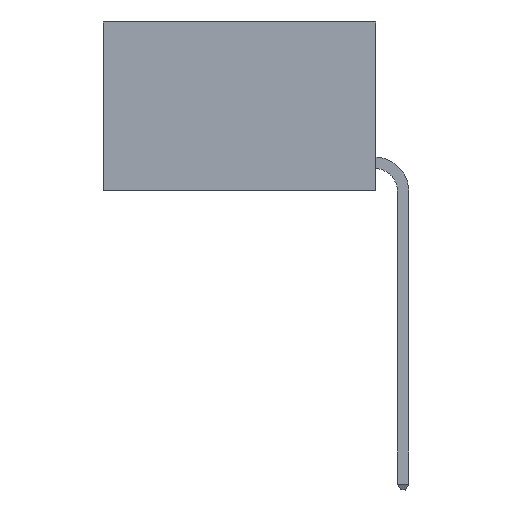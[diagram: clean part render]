
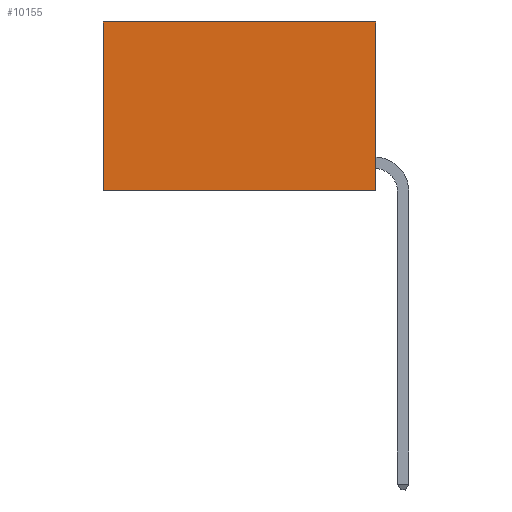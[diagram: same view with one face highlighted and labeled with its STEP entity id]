
A CAD part, left-side view. The second image highlights one B-rep face of the part: STEP entity #10155.
In plain terms, the highlighted planar face has unit normal (-1, 0, 0).
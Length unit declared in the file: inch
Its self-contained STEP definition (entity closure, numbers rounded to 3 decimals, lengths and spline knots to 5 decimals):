
#822 = DIRECTION ( 'NONE',  ( 0., 0., -1. ) ) ;
#2356 = PLANE ( 'NONE',  #9571 ) ;
#2673 = EDGE_CURVE ( 'NONE', #13012, #13319, #8842, .T. ) ;
#3315 = CARTESIAN_POINT ( 'NONE',  ( 0.2625, 0., -0.37 ) ) ;
#3346 = DIRECTION ( 'NONE',  ( 0., 0., -1. ) ) ;
#5796 = CARTESIAN_POINT ( 'NONE',  ( 0.2625, 0., 0. ) ) ;
#5929 = VECTOR ( 'NONE', #3346, 39.37008 ) ;
#6396 = CARTESIAN_POINT ( 'NONE',  ( 0.2625, 0.6, 0. ) ) ;
#6825 = EDGE_LOOP ( 'NONE', ( #9311, #16320, #16991, #8579 ) ) ;
#6962 = CARTESIAN_POINT ( 'NONE',  ( 0.2625, 0., 0. ) ) ;
#7370 = VECTOR ( 'NONE', #822, 39.37008 ) ;
#7452 = DIRECTION ( 'NONE',  ( 0., 1., 0. ) ) ;
#7479 = DIRECTION ( 'NONE',  ( 0., 0., -1. ) ) ;
#8579 = ORIENTED_EDGE ( 'NONE', *, *, #17465, .T. ) ;
#8842 = LINE ( 'NONE', #14641, #17308 ) ;
#9311 = ORIENTED_EDGE ( 'NONE', *, *, #16214, .T. ) ;
#9571 = AXIS2_PLACEMENT_3D ( 'NONE', #5796, #17603, #7479 ) ;
#10155 = ADVANCED_FACE ( 'NONE', ( #21422 ), #2356, .F. ) ;
#10308 = DIRECTION ( 'NONE',  ( 0., 1., 0. ) ) ;
#10760 = CARTESIAN_POINT ( 'NONE',  ( 0.2625, 0.6, -0.37 ) ) ;
#10913 = LINE ( 'NONE', #13501, #5929 ) ;
#11003 = CARTESIAN_POINT ( 'NONE',  ( 0.2625, 0., 0. ) ) ;
#11380 = VECTOR ( 'NONE', #10308, 39.37008 ) ;
#13012 = VERTEX_POINT ( 'NONE', #3315 ) ;
#13319 = VERTEX_POINT ( 'NONE', #10760 ) ;
#13501 = CARTESIAN_POINT ( 'NONE',  ( 0.2625, 0.6, 0. ) ) ;
#13583 = VERTEX_POINT ( 'NONE', #19831 ) ;
#14641 = CARTESIAN_POINT ( 'NONE',  ( 0.2625, 0., -0.37 ) ) ;
#16214 = EDGE_CURVE ( 'NONE', #20518, #13319, #10913, .T. ) ;
#16320 = ORIENTED_EDGE ( 'NONE', *, *, #2673, .F. ) ;
#16378 = LINE ( 'NONE', #11003, #7370 ) ;
#16991 = ORIENTED_EDGE ( 'NONE', *, *, #19161, .F. ) ;
#17308 = VECTOR ( 'NONE', #7452, 39.37008 ) ;
#17465 = EDGE_CURVE ( 'NONE', #13583, #20518, #20370, .T. ) ;
#17603 = DIRECTION ( 'NONE',  ( 1., 0., 0. ) ) ;
#19161 = EDGE_CURVE ( 'NONE', #13583, #13012, #16378, .T. ) ;
#19831 = CARTESIAN_POINT ( 'NONE',  ( 0.2625, 0., 0. ) ) ;
#20370 = LINE ( 'NONE', #6962, #11380 ) ;
#20518 = VERTEX_POINT ( 'NONE', #6396 ) ;
#21422 = FACE_OUTER_BOUND ( 'NONE', #6825, .T. ) ;
